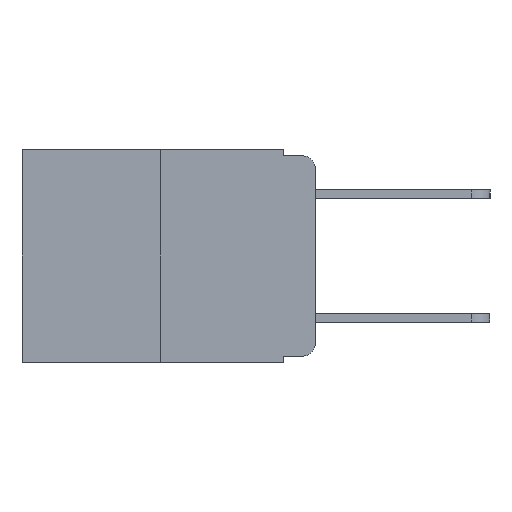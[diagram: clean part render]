
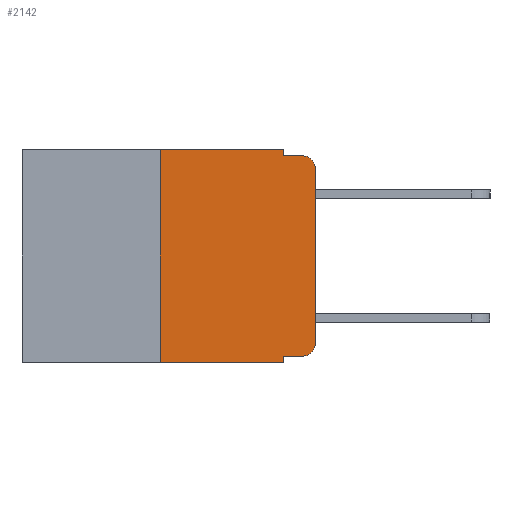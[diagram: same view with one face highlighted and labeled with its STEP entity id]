
A CAD part, left-side view. The second image highlights one B-rep face of the part: STEP entity #2142.
In plain terms, the highlighted planar face has unit normal (-1, 0, 0).
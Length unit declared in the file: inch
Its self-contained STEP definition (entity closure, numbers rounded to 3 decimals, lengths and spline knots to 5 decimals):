
#12 = VERTEX_POINT ( 'NONE', #6496 ) ;
#290 = CARTESIAN_POINT ( 'NONE',  ( 0., 0.051, -0.01 ) ) ;
#532 = CIRCLE ( 'NONE', #9942, 0.02 ) ;
#647 = LINE ( 'NONE', #10041, #10564 ) ;
#692 = EDGE_CURVE ( 'NONE', #9805, #12, #532, .T. ) ;
#850 = DIRECTION ( 'NONE',  ( 0., -1., 0. ) ) ;
#1008 = DIRECTION ( 'NONE',  ( 0., 0., -1. ) ) ;
#1028 = CARTESIAN_POINT ( 'NONE',  ( 0., 0.02, -0.333 ) ) ;
#1384 = LINE ( 'NONE', #5861, #6733 ) ;
#1674 = EDGE_CURVE ( 'NONE', #11963, #4214, #7098, .T. ) ;
#1782 = CARTESIAN_POINT ( 'NONE',  ( 0., 0.473, 0. ) ) ;
#2100 = ORIENTED_EDGE ( 'NONE', *, *, #4546, .F. ) ;
#2142 = ADVANCED_FACE ( 'NONE', ( #8640 ), #2784, .F. ) ;
#2290 = DIRECTION ( 'NONE',  ( 0., -1., 0. ) ) ;
#2298 = VERTEX_POINT ( 'NONE', #3545 ) ;
#2392 = CARTESIAN_POINT ( 'NONE',  ( 0., 0.051, -0.333 ) ) ;
#2498 = VERTEX_POINT ( 'NONE', #7563 ) ;
#2661 = VERTEX_POINT ( 'NONE', #2688 ) ;
#2688 = CARTESIAN_POINT ( 'NONE',  ( 0., 0., -0.03 ) ) ;
#2691 = EDGE_CURVE ( 'NONE', #10167, #2298, #10880, .T. ) ;
#2758 = ORIENTED_EDGE ( 'NONE', *, *, #11557, .F. ) ;
#2784 = PLANE ( 'NONE',  #9499 ) ;
#3155 = EDGE_CURVE ( 'NONE', #2661, #4204, #6460, .T. ) ;
#3217 = CARTESIAN_POINT ( 'NONE',  ( 0., 0.473, 0. ) ) ;
#3372 = VECTOR ( 'NONE', #9886, 39.37008 ) ;
#3408 = EDGE_CURVE ( 'NONE', #12, #2661, #647, .T. ) ;
#3482 = LINE ( 'NONE', #7260, #8362 ) ;
#3545 = CARTESIAN_POINT ( 'NONE',  ( 0., 0.051, -0.343 ) ) ;
#3596 = ORIENTED_EDGE ( 'NONE', *, *, #2691, .F. ) ;
#3850 = EDGE_CURVE ( 'NONE', #10167, #9805, #3482, .T. ) ;
#4082 = CARTESIAN_POINT ( 'NONE',  ( 0., 0.02, -0.01 ) ) ;
#4199 = VECTOR ( 'NONE', #7305, 39.37008 ) ;
#4204 = VERTEX_POINT ( 'NONE', #4082 ) ;
#4214 = VERTEX_POINT ( 'NONE', #7987 ) ;
#4259 = ORIENTED_EDGE ( 'NONE', *, *, #3850, .T. ) ;
#4466 = CARTESIAN_POINT ( 'NONE',  ( 0., 0.051, 0. ) ) ;
#4545 = EDGE_CURVE ( 'NONE', #2498, #2298, #1384, .T. ) ;
#4546 = EDGE_CURVE ( 'NONE', #5362, #4204, #9150, .T. ) ;
#5362 = VERTEX_POINT ( 'NONE', #290 ) ;
#5704 = EDGE_LOOP ( 'NONE', ( #10783, #9242, #2100, #2758, #10351, #8842, #5921, #3596, #4259, #7459 ) ) ;
#5861 = CARTESIAN_POINT ( 'NONE',  ( 0., 0.473, -0.343 ) ) ;
#5900 = CARTESIAN_POINT ( 'NONE',  ( 0., 0.02, -0.03 ) ) ;
#5921 = ORIENTED_EDGE ( 'NONE', *, *, #4545, .T. ) ;
#6460 = CIRCLE ( 'NONE', #7965, 0.02 ) ;
#6496 = CARTESIAN_POINT ( 'NONE',  ( 0., 0., -0.313 ) ) ;
#6733 = VECTOR ( 'NONE', #12173, 39.37008 ) ;
#6814 = LINE ( 'NONE', #9369, #11581 ) ;
#6903 = DIRECTION ( 'NONE',  ( 0., 0., -1. ) ) ;
#7042 = DIRECTION ( 'NONE',  ( 0., 0., -1. ) ) ;
#7098 = LINE ( 'NONE', #3217, #8925 ) ;
#7260 = CARTESIAN_POINT ( 'NONE',  ( 0., 0.051, -0.333 ) ) ;
#7305 = DIRECTION ( 'NONE',  ( 0., 0., 1. ) ) ;
#7459 = ORIENTED_EDGE ( 'NONE', *, *, #692, .T. ) ;
#7563 = CARTESIAN_POINT ( 'NONE',  ( 0., 0.25, -0.343 ) ) ;
#7965 = AXIS2_PLACEMENT_3D ( 'NONE', #5900, #12206, #6903 ) ;
#7987 = CARTESIAN_POINT ( 'NONE',  ( 0., 0.051, 0. ) ) ;
#8189 = DIRECTION ( 'NONE',  ( 0., -1., 0. ) ) ;
#8331 = DIRECTION ( 'NONE',  ( 1., 0., 0. ) ) ;
#8362 = VECTOR ( 'NONE', #8189, 39.37008 ) ;
#8640 = FACE_OUTER_BOUND ( 'NONE', #5704, .T. ) ;
#8662 = CARTESIAN_POINT ( 'NONE',  ( 0., 0.051, -0.01 ) ) ;
#8842 = ORIENTED_EDGE ( 'NONE', *, *, #12115, .F. ) ;
#8873 = VECTOR ( 'NONE', #850, 39.37008 ) ;
#8925 = VECTOR ( 'NONE', #2290, 39.37008 ) ;
#9052 = CARTESIAN_POINT ( 'NONE',  ( 0., 0.25, 0. ) ) ;
#9145 = DIRECTION ( 'NONE',  ( 0., 0., 1. ) ) ;
#9150 = LINE ( 'NONE', #8662, #8873 ) ;
#9204 = LINE ( 'NONE', #9052, #4199 ) ;
#9242 = ORIENTED_EDGE ( 'NONE', *, *, #3155, .T. ) ;
#9369 = CARTESIAN_POINT ( 'NONE',  ( 0., 0.051, 0. ) ) ;
#9499 = AXIS2_PLACEMENT_3D ( 'NONE', #1782, #8331, #1008 ) ;
#9504 = DIRECTION ( 'NONE',  ( -1., 0., 0. ) ) ;
#9532 = CARTESIAN_POINT ( 'NONE',  ( 0., 0.02, -0.313 ) ) ;
#9805 = VERTEX_POINT ( 'NONE', #1028 ) ;
#9886 = DIRECTION ( 'NONE',  ( 0., 0., -1. ) ) ;
#9942 = AXIS2_PLACEMENT_3D ( 'NONE', #9532, #9504, #7042 ) ;
#10041 = CARTESIAN_POINT ( 'NONE',  ( 0., 0., 0. ) ) ;
#10167 = VERTEX_POINT ( 'NONE', #2392 ) ;
#10351 = ORIENTED_EDGE ( 'NONE', *, *, #1674, .F. ) ;
#10564 = VECTOR ( 'NONE', #9145, 39.37008 ) ;
#10683 = CARTESIAN_POINT ( 'NONE',  ( 0., 0.25, 0. ) ) ;
#10783 = ORIENTED_EDGE ( 'NONE', *, *, #3408, .T. ) ;
#10880 = LINE ( 'NONE', #4466, #3372 ) ;
#11557 = EDGE_CURVE ( 'NONE', #4214, #5362, #6814, .T. ) ;
#11581 = VECTOR ( 'NONE', #12015, 39.37008 ) ;
#11963 = VERTEX_POINT ( 'NONE', #10683 ) ;
#12015 = DIRECTION ( 'NONE',  ( 0., 0., -1. ) ) ;
#12115 = EDGE_CURVE ( 'NONE', #2498, #11963, #9204, .T. ) ;
#12173 = DIRECTION ( 'NONE',  ( 0., -1., 0. ) ) ;
#12206 = DIRECTION ( 'NONE',  ( -1., 0., 0. ) ) ;
